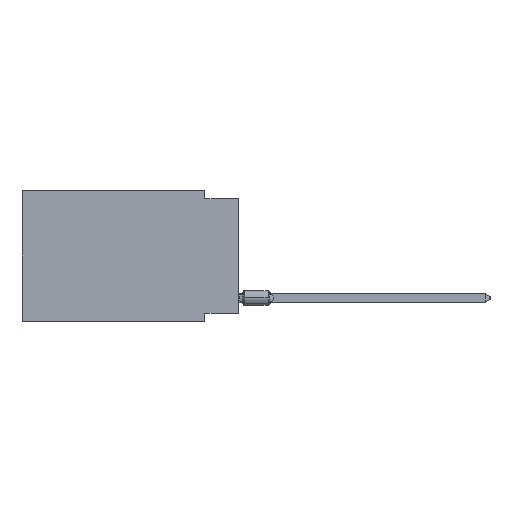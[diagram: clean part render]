
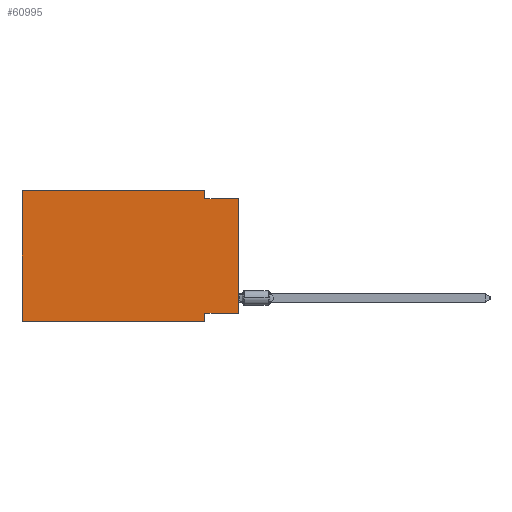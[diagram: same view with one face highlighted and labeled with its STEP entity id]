
A CAD part, left-side view. The second image highlights one B-rep face of the part: STEP entity #60995.
In plain terms, the highlighted planar face has unit normal (-1, 0, 0).
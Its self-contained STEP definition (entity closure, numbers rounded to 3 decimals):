
#572 = VERTEX_POINT ( 'NONE', #50994 ) ;
#906 = DIRECTION ( 'NONE',  ( 0., -1., 0. ) ) ;
#1307 = CARTESIAN_POINT ( 'NONE',  ( 0., 16.383, 0. ) ) ;
#1847 = VECTOR ( 'NONE', #44717, 1000. ) ;
#2025 = CARTESIAN_POINT ( 'NONE',  ( 0., 16.383, -9.906 ) ) ;
#3616 = CARTESIAN_POINT ( 'NONE',  ( 0., 2.54, -0.635 ) ) ;
#4974 = VERTEX_POINT ( 'NONE', #46742 ) ;
#6694 = VERTEX_POINT ( 'NONE', #48162 ) ;
#7182 = EDGE_CURVE ( 'NONE', #22979, #35482, #44432, .T. ) ;
#8969 = CARTESIAN_POINT ( 'NONE',  ( 0., 16.383, 0. ) ) ;
#9133 = EDGE_CURVE ( 'NONE', #50496, #4974, #47960, .T. ) ;
#10931 = VECTOR ( 'NONE', #906, 1000. ) ;
#13659 = LINE ( 'NONE', #8969, #27082 ) ;
#13845 = CARTESIAN_POINT ( 'NONE',  ( 0., 0., -9.271 ) ) ;
#15260 = EDGE_CURVE ( 'NONE', #4974, #22979, #53755, .T. ) ;
#16701 = VECTOR ( 'NONE', #38686, 1000. ) ;
#16990 = CARTESIAN_POINT ( 'NONE',  ( 0., 16.383, -9.906 ) ) ;
#18250 = DIRECTION ( 'NONE',  ( 0., 1., 0. ) ) ;
#19494 = DIRECTION ( 'NONE',  ( 1., 0., 0. ) ) ;
#19553 = CARTESIAN_POINT ( 'NONE',  ( 0., 2.54, 0. ) ) ;
#20035 = ORIENTED_EDGE ( 'NONE', *, *, #9133, .F. ) ;
#20326 = EDGE_CURVE ( 'NONE', #53512, #6694, #33305, .T. ) ;
#21660 = EDGE_LOOP ( 'NONE', ( #55915, #27037, #31693, #20035, #59776, #37015, #48272, #28248 ) ) ;
#22979 = VERTEX_POINT ( 'NONE', #3616 ) ;
#24419 = VECTOR ( 'NONE', #18250, 1000. ) ;
#24455 = CARTESIAN_POINT ( 'NONE',  ( 0., 0., -9.271 ) ) ;
#25851 = LINE ( 'NONE', #2025, #61808 ) ;
#27037 = ORIENTED_EDGE ( 'NONE', *, *, #7182, .F. ) ;
#27082 = VECTOR ( 'NONE', #46608, 1000. ) ;
#28248 = ORIENTED_EDGE ( 'NONE', *, *, #20326, .F. ) ;
#30993 = VECTOR ( 'NONE', #54407, 1000. ) ;
#31693 = ORIENTED_EDGE ( 'NONE', *, *, #15260, .F. ) ;
#32151 = VECTOR ( 'NONE', #49686, 1000. ) ;
#33305 = LINE ( 'NONE', #13845, #24419 ) ;
#34562 = PLANE ( 'NONE',  #49238 ) ;
#34771 = CARTESIAN_POINT ( 'NONE',  ( 0., 16.383, 0. ) ) ;
#34860 = DIRECTION ( 'NONE',  ( 0., 0., -1. ) ) ;
#35262 = CARTESIAN_POINT ( 'NONE',  ( 0., 0., 0. ) ) ;
#35482 = VERTEX_POINT ( 'NONE', #38412 ) ;
#35869 = CARTESIAN_POINT ( 'NONE',  ( 0., 2.54, -9.906 ) ) ;
#37015 = ORIENTED_EDGE ( 'NONE', *, *, #55529, .T. ) ;
#37569 = EDGE_CURVE ( 'NONE', #6694, #572, #60410, .T. ) ;
#37572 = CARTESIAN_POINT ( 'NONE',  ( 0., 16.383, 0. ) ) ;
#38412 = CARTESIAN_POINT ( 'NONE',  ( 0., 0., -0.635 ) ) ;
#38686 = DIRECTION ( 'NONE',  ( 0., 0., -1. ) ) ;
#38710 = LINE ( 'NONE', #35262, #30993 ) ;
#39224 = VERTEX_POINT ( 'NONE', #16990 ) ;
#39416 = CARTESIAN_POINT ( 'NONE',  ( 0., 0., -0.635 ) ) ;
#40878 = EDGE_CURVE ( 'NONE', #39224, #50496, #13659, .T. ) ;
#44432 = LINE ( 'NONE', #39416, #1847 ) ;
#44717 = DIRECTION ( 'NONE',  ( 0., -1., 0. ) ) ;
#45337 = EDGE_CURVE ( 'NONE', #53512, #35482, #38710, .T. ) ;
#46608 = DIRECTION ( 'NONE',  ( 0., 0., 1. ) ) ;
#46742 = CARTESIAN_POINT ( 'NONE',  ( 0., 2.54, 0. ) ) ;
#47960 = LINE ( 'NONE', #34771, #10931 ) ;
#48162 = CARTESIAN_POINT ( 'NONE',  ( 0., 2.54, -9.271 ) ) ;
#48272 = ORIENTED_EDGE ( 'NONE', *, *, #37569, .F. ) ;
#49238 = AXIS2_PLACEMENT_3D ( 'NONE', #1307, #19494, #34860 ) ;
#49307 = FACE_OUTER_BOUND ( 'NONE', #21660, .T. ) ;
#49686 = DIRECTION ( 'NONE',  ( 0., 0., -1. ) ) ;
#50496 = VERTEX_POINT ( 'NONE', #37572 ) ;
#50994 = CARTESIAN_POINT ( 'NONE',  ( 0., 2.54, -9.906 ) ) ;
#53512 = VERTEX_POINT ( 'NONE', #24455 ) ;
#53755 = LINE ( 'NONE', #19553, #16701 ) ;
#54407 = DIRECTION ( 'NONE',  ( 0., 0., 1. ) ) ;
#55529 = EDGE_CURVE ( 'NONE', #39224, #572, #25851, .T. ) ;
#55915 = ORIENTED_EDGE ( 'NONE', *, *, #45337, .T. ) ;
#59764 = DIRECTION ( 'NONE',  ( 0., -1., 0. ) ) ;
#59776 = ORIENTED_EDGE ( 'NONE', *, *, #40878, .F. ) ;
#60410 = LINE ( 'NONE', #35869, #32151 ) ;
#60995 = ADVANCED_FACE ( 'NONE', ( #49307 ), #34562, .F. ) ;
#61808 = VECTOR ( 'NONE', #59764, 1000. ) ;
